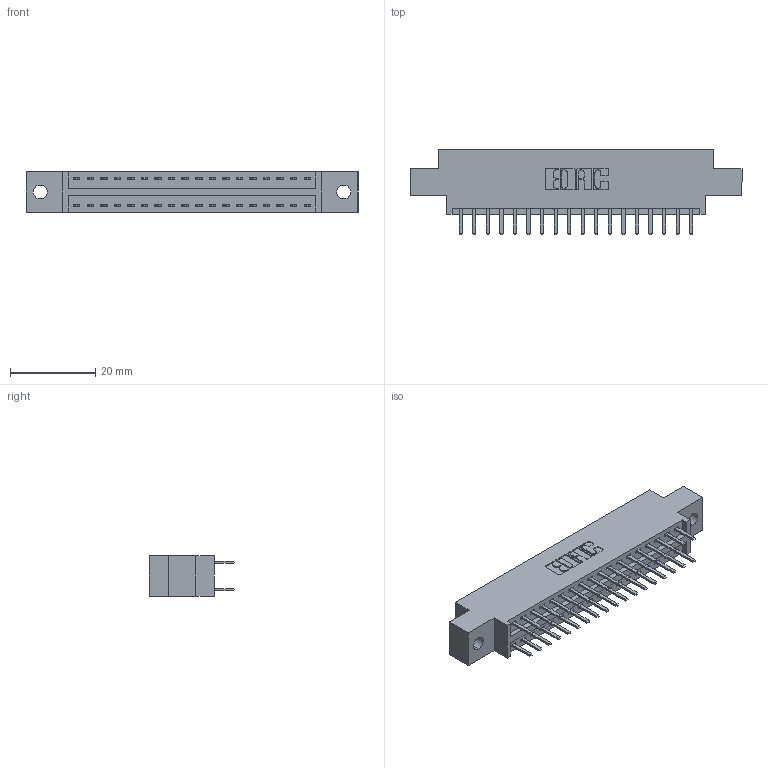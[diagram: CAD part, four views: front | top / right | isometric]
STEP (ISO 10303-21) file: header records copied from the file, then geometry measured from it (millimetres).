
FILE_DESCRIPTION (( 'STEP AP203' ), '1' );
FILE_NAME ('346-036-520-802.STEP', '2022-05-19T21:00:06', ( '' ), ( '' ), 'SwSTEP 2.0', 'SolidWorks 2020', '' );
FILE_SCHEMA (( 'CONFIG_CONTROL_DESIGN' ));
Length unit declared in the file: inch
Products named in the file (3): 346 Part_0.170 Offset - 0.128 Dia; 346-036-520-802; 345-292-001_345-293-120
Assembly tree (37 placements, depth 2):
  346-036-520-802
    346 Part_0.170 Offset - 0.128 Dia
    345-292-001_345-293-120  x36
Bounding box: 77.72 x 20.02 x 9.4 mm (x, y, z)
Volume: 7185.5 mm3; surface area: 9373.1 mm2
Topology: 37 solids, 37 shells, 2142 faces, 6209 edges, 4042 vertices
Faces by surface type: plane 1412, cylinder 730
Entity records: 15227 total; most frequent: CARTESIAN_POINT 2556, ORIENTED_EDGE 2478, DIRECTION 2291, EDGE_CURVE 1239, VECTOR 1031, LINE 1031, VERTEX_POINT 822, AXIS2_PLACEMENT_3D 630
